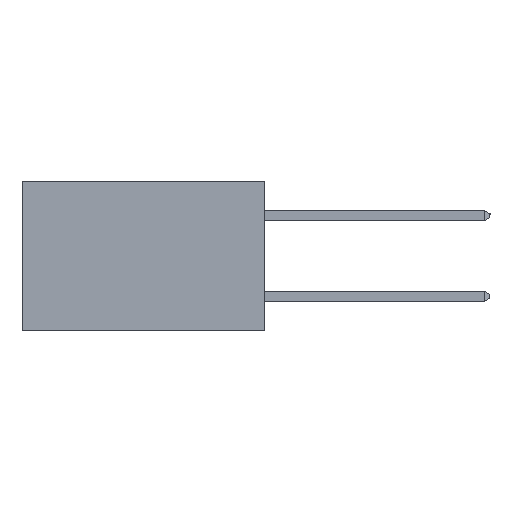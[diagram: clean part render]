
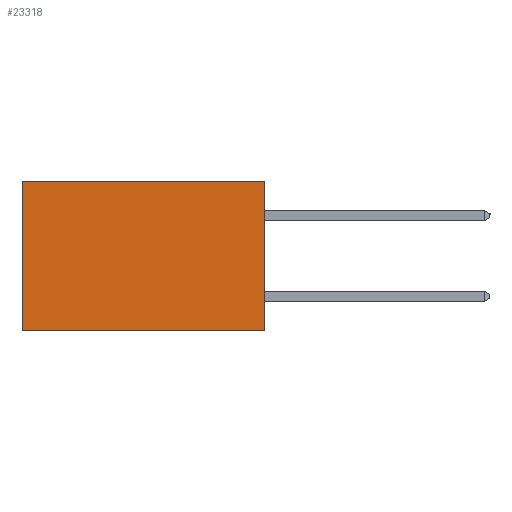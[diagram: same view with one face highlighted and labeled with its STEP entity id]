
A CAD part, left-side view. The second image highlights one B-rep face of the part: STEP entity #23318.
In plain terms, the highlighted planar face has unit normal (-1, 0, 0).
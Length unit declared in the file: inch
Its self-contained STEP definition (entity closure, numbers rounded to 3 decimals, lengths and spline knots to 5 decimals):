
#2044 = DIRECTION ( 'NONE',  ( 0., 0., -1. ) ) ;
#3315 = EDGE_CURVE ( 'NONE', #17159, #21869, #20333, .T. ) ;
#3478 = EDGE_CURVE ( 'NONE', #21820, #17159, #8931, .T. ) ;
#3583 = PLANE ( 'NONE',  #9247 ) ;
#3820 = DIRECTION ( 'NONE',  ( 1., 0., 0. ) ) ;
#4169 = ORIENTED_EDGE ( 'NONE', *, *, #3478, .F. ) ;
#4721 = VECTOR ( 'NONE', #21164, 39.37008 ) ;
#5053 = VECTOR ( 'NONE', #11107, 39.37008 ) ;
#5854 = LINE ( 'NONE', #16476, #6299 ) ;
#6022 = VERTEX_POINT ( 'NONE', #11996 ) ;
#6299 = VECTOR ( 'NONE', #2044, 39.37008 ) ;
#7512 = ORIENTED_EDGE ( 'NONE', *, *, #12966, .T. ) ;
#8475 = ORIENTED_EDGE ( 'NONE', *, *, #3315, .F. ) ;
#8570 = CARTESIAN_POINT ( 'NONE',  ( 0.2615, 0., -0.37 ) ) ;
#8931 = LINE ( 'NONE', #8570, #22641 ) ;
#9247 = AXIS2_PLACEMENT_3D ( 'NONE', #14657, #3820, #21864 ) ;
#10229 = CARTESIAN_POINT ( 'NONE',  ( 0.2615, 0., -0.37 ) ) ;
#11107 = DIRECTION ( 'NONE',  ( 0., 1., 0. ) ) ;
#11251 = EDGE_CURVE ( 'NONE', #21820, #6022, #21278, .T. ) ;
#11996 = CARTESIAN_POINT ( 'NONE',  ( 0.2615, 0.6, 0. ) ) ;
#12966 = EDGE_CURVE ( 'NONE', #6022, #21869, #5854, .T. ) ;
#14386 = ORIENTED_EDGE ( 'NONE', *, *, #11251, .T. ) ;
#14472 = DIRECTION ( 'NONE',  ( 0., 0., -1. ) ) ;
#14657 = CARTESIAN_POINT ( 'NONE',  ( 0.2615, 0., -0.37 ) ) ;
#16476 = CARTESIAN_POINT ( 'NONE',  ( 0.2615, 0.6, -0.37 ) ) ;
#17159 = VERTEX_POINT ( 'NONE', #10229 ) ;
#18433 = CARTESIAN_POINT ( 'NONE',  ( 0.2615, 0., -0.37 ) ) ;
#19952 = EDGE_LOOP ( 'NONE', ( #7512, #8475, #4169, #14386 ) ) ;
#20152 = FACE_OUTER_BOUND ( 'NONE', #19952, .T. ) ;
#20190 = CARTESIAN_POINT ( 'NONE',  ( 0.2615, 0.6, -0.37 ) ) ;
#20333 = LINE ( 'NONE', #18433, #5053 ) ;
#21164 = DIRECTION ( 'NONE',  ( 0., 1., 0. ) ) ;
#21278 = LINE ( 'NONE', #23086, #4721 ) ;
#21415 = CARTESIAN_POINT ( 'NONE',  ( 0.2615, 0., 0. ) ) ;
#21820 = VERTEX_POINT ( 'NONE', #21415 ) ;
#21864 = DIRECTION ( 'NONE',  ( 0., 0., -1. ) ) ;
#21869 = VERTEX_POINT ( 'NONE', #20190 ) ;
#22641 = VECTOR ( 'NONE', #14472, 39.37008 ) ;
#23086 = CARTESIAN_POINT ( 'NONE',  ( 0.2615, 0., 0. ) ) ;
#23318 = ADVANCED_FACE ( 'NONE', ( #20152 ), #3583, .F. ) ;
